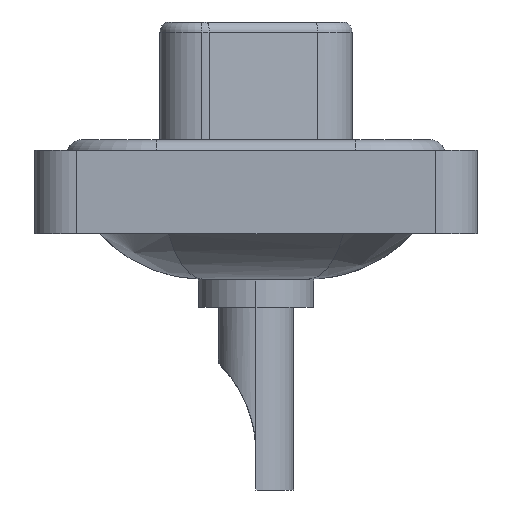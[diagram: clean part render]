
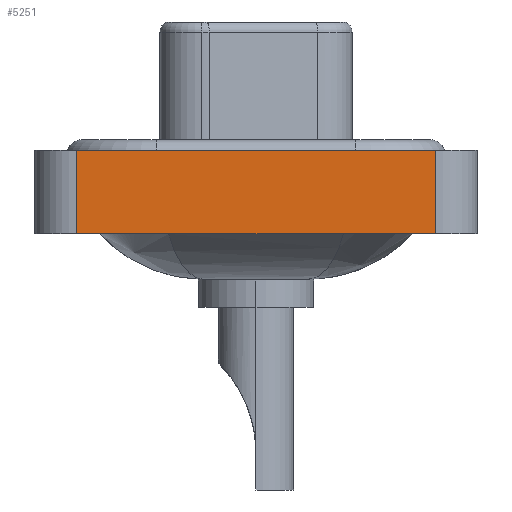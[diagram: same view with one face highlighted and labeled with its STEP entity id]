
A CAD part, left-side view. The second image highlights one B-rep face of the part: STEP entity #5251.
In plain terms, the highlighted planar face has unit normal (-1, 0, 0).
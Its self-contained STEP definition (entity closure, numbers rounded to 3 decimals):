
#301 = EDGE_CURVE ( 'NONE', #15278, #7705, #6691, .T. ) ;
#1038 = EDGE_LOOP ( 'NONE', ( #14414, #11493, #2173, #14393 ) ) ;
#1101 = EDGE_CURVE ( 'NONE', #7705, #16238, #10004, .T. ) ;
#1180 = DIRECTION ( 'NONE',  ( 0., 0., 1. ) ) ;
#1310 = VECTOR ( 'NONE', #10182, 1000. ) ;
#1645 = DIRECTION ( 'NONE',  ( 0., -1., 0. ) ) ;
#2173 = ORIENTED_EDGE ( 'NONE', *, *, #6264, .F. ) ;
#2999 = EDGE_CURVE ( 'NONE', #8374, #16238, #6168, .T. ) ;
#3229 = PLANE ( 'NONE',  #6749 ) ;
#5110 = CARTESIAN_POINT ( 'NONE',  ( -7.3, -8.55, -3.6 ) ) ;
#5251 = ADVANCED_FACE ( 'NONE', ( #12470 ), #3229, .T. ) ;
#5419 = VECTOR ( 'NONE', #1645, 1000. ) ;
#5778 = CARTESIAN_POINT ( 'NONE',  ( -7.3, -8.55, -3.6 ) ) ;
#6031 = DIRECTION ( 'NONE',  ( 0., 0., 1. ) ) ;
#6168 = LINE ( 'NONE', #12873, #16406 ) ;
#6264 = EDGE_CURVE ( 'NONE', #15278, #8374, #9127, .T. ) ;
#6505 = DIRECTION ( 'NONE',  ( 0., -1., 0. ) ) ;
#6691 = LINE ( 'NONE', #9510, #5419 ) ;
#6749 = AXIS2_PLACEMENT_3D ( 'NONE', #5778, #11027, #6031 ) ;
#7705 = VERTEX_POINT ( 'NONE', #9867 ) ;
#8374 = VERTEX_POINT ( 'NONE', #10755 ) ;
#8955 = VECTOR ( 'NONE', #1180, 1000. ) ;
#8957 = CARTESIAN_POINT ( 'NONE',  ( -7.3, 8.55, -3.6 ) ) ;
#9127 = LINE ( 'NONE', #8957, #8955 ) ;
#9510 = CARTESIAN_POINT ( 'NONE',  ( -7.3, -8.55, -3.6 ) ) ;
#9867 = CARTESIAN_POINT ( 'NONE',  ( -7.3, -8.55, -3.6 ) ) ;
#10004 = LINE ( 'NONE', #5110, #1310 ) ;
#10182 = DIRECTION ( 'NONE',  ( 0., 0., 1. ) ) ;
#10755 = CARTESIAN_POINT ( 'NONE',  ( -7.3, 8.55, 0.4 ) ) ;
#11027 = DIRECTION ( 'NONE',  ( -1., 0., 0. ) ) ;
#11493 = ORIENTED_EDGE ( 'NONE', *, *, #2999, .F. ) ;
#11937 = CARTESIAN_POINT ( 'NONE',  ( -7.3, -8.55, 0.4 ) ) ;
#12470 = FACE_OUTER_BOUND ( 'NONE', #1038, .T. ) ;
#12873 = CARTESIAN_POINT ( 'NONE',  ( -7.3, -8.55, 0.4 ) ) ;
#12936 = CARTESIAN_POINT ( 'NONE',  ( -7.3, 8.55, -3.6 ) ) ;
#14393 = ORIENTED_EDGE ( 'NONE', *, *, #301, .T. ) ;
#14414 = ORIENTED_EDGE ( 'NONE', *, *, #1101, .T. ) ;
#15278 = VERTEX_POINT ( 'NONE', #12936 ) ;
#16238 = VERTEX_POINT ( 'NONE', #11937 ) ;
#16406 = VECTOR ( 'NONE', #6505, 1000. ) ;
